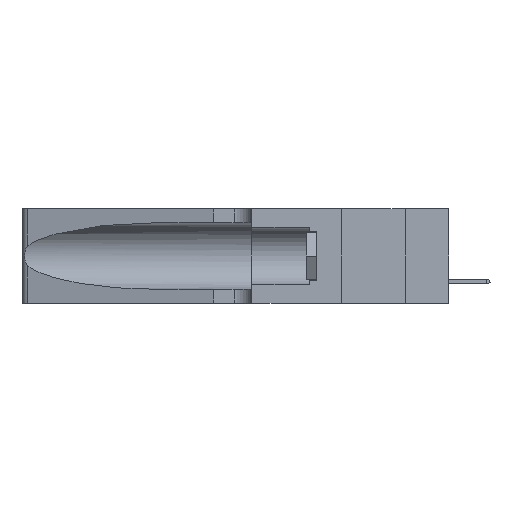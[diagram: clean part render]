
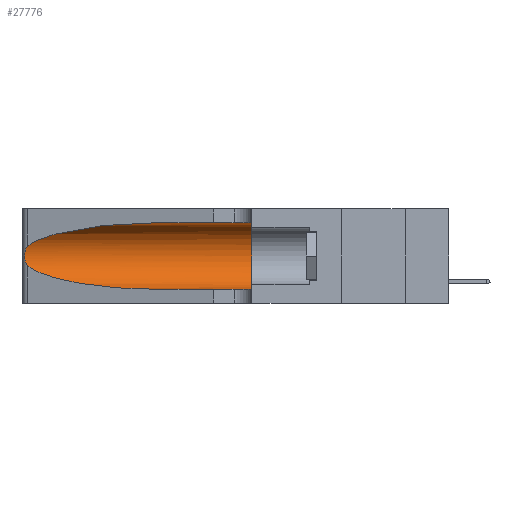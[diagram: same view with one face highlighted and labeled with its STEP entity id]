
A CAD part, left-side view. The second image highlights one B-rep face of the part: STEP entity #27776.
In plain terms, the highlighted cylindrical face has radius 3.308 mm (diameter 6.617 mm), a partial arc.
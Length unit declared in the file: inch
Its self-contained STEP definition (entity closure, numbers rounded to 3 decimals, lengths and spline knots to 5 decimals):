
#240 = VERTEX_POINT ( 'NONE', #22419 ) ;
#779 = CARTESIAN_POINT ( 'NONE',  ( 0.1305, 1.61858, 0.31525 ) ) ;
#993 = LINE ( 'NONE', #779, #8944 ) ;
#1124 = DIRECTION ( 'NONE',  ( 0., -1., 0. ) ) ;
#1543 = DIRECTION ( 'NONE',  ( 0., 0., 1. ) ) ;
#1784 = CARTESIAN_POINT ( 'NONE',  ( 0.25789, 1.23486, 0.15765 ) ) ;
#2504 = AXIS2_PLACEMENT_3D ( 'NONE', #30883, #9723, #1543 ) ;
#3566 = VERTEX_POINT ( 'NONE', #3942 ) ;
#3942 = CARTESIAN_POINT ( 'NONE',  ( 0.1305, 0.35, 0.05475 ) ) ;
#4253 = CARTESIAN_POINT ( 'NONE',  ( 0.25639, 1.23184, 0.21858 ) ) ;
#4549 = CARTESIAN_POINT ( 'NONE',  ( 0.18966, 0.96281, 0.31525 ) ) ;
#5042 = CARTESIAN_POINT ( 'NONE',  ( 0.2373, 1.15595, 0.08982 ) ) ;
#5428 = EDGE_CURVE ( 'NONE', #18067, #3566, #24555, .T. ) ;
#7059 = VERTEX_POINT ( 'NONE', #33663 ) ;
#8215 =( BOUNDED_CURVE ( )  B_SPLINE_CURVE ( 3, ( #15352, #5042, #10431, #34454 ),
 .UNSPECIFIED., .F., .T. ) 
 B_SPLINE_CURVE_WITH_KNOTS ( ( 4, 4 ),
 ( 3.44316, 4.71239 ),
 .UNSPECIFIED. ) 
 CURVE ( )  GEOMETRIC_REPRESENTATION_ITEM ( )  RATIONAL_B_SPLINE_CURVE ( ( 1., 0.87, 0.87, 1. ) ) 
 REPRESENTATION_ITEM ( '' )  );
#8944 = VECTOR ( 'NONE', #22299, 39.37008 ) ;
#9069 = DIRECTION ( 'NONE',  ( 0., 0., -1. ) ) ;
#9390 = CARTESIAN_POINT ( 'NONE',  ( 0.25854, 1.2359, 0.20912 ) ) ;
#9656 = DIRECTION ( 'NONE',  ( 0., -1., 0. ) ) ;
#9689 = CARTESIAN_POINT ( 'NONE',  ( 0.2373, 1.15595, 0.28018 ) ) ;
#9723 = DIRECTION ( 'NONE',  ( 0., 1., 0. ) ) ;
#9742 = CARTESIAN_POINT ( 'NONE',  ( 0.25639, 1.23186, 0.15144 ) ) ;
#9858 = CARTESIAN_POINT ( 'NONE',  ( 0.25487, 1.22718, 0.14631 ) ) ;
#9927 = CARTESIAN_POINT ( 'NONE',  ( 0.25487, 1.22718, 0.22369 ) ) ;
#10431 = CARTESIAN_POINT ( 'NONE',  ( 0.18966, 0.96281, 0.05475 ) ) ;
#10517 = ORIENTED_EDGE ( 'NONE', *, *, #25509, .T. ) ;
#11369 = CYLINDRICAL_SURFACE ( 'NONE', #30823, 0.13025 ) ;
#11950 = EDGE_CURVE ( 'NONE', #7059, #240, #20709, .T. ) ;
#12295 = CARTESIAN_POINT ( 'NONE',  ( 0.1305, 0.72297, 0.31525 ) ) ;
#12446 = ORIENTED_EDGE ( 'NONE', *, *, #11950, .T. ) ;
#12728 = VERTEX_POINT ( 'NONE', #17952 ) ;
#14496 = EDGE_CURVE ( 'NONE', #12728, #7059, #25820, .T. ) ;
#15352 = CARTESIAN_POINT ( 'NONE',  ( 0.25487, 1.22718, 0.14631 ) ) ;
#16050 = ORIENTED_EDGE ( 'NONE', *, *, #5428, .F. ) ;
#16152 = ORIENTED_EDGE ( 'NONE', *, *, #25764, .F. ) ;
#17034 = CARTESIAN_POINT ( 'NONE',  ( 0.1305, 1.61858, 0.185 ) ) ;
#17288 = ORIENTED_EDGE ( 'NONE', *, *, #18396, .T. ) ;
#17952 = CARTESIAN_POINT ( 'NONE',  ( 0.1305, 0.72297, 0.31525 ) ) ;
#18067 = VERTEX_POINT ( 'NONE', #29115 ) ;
#18165 = LINE ( 'NONE', #33691, #22287 ) ;
#18396 = EDGE_CURVE ( 'NONE', #24721, #3566, #18165, .T. ) ;
#20376 = CARTESIAN_POINT ( 'NONE',  ( 0.25487, 1.22718, 0.22369 ) ) ;
#20709 = B_SPLINE_CURVE_WITH_KNOTS ( 'NONE', 3,
 ( #20376, #25865, #4253, #25505, #9390, #23046, #28556, #25749, #22933, #25383, #1784, #9742, #28082, #9858 ),
 .UNSPECIFIED., .F., .F.,
 ( 4, 2, 2, 2, 2, 2, 4 ),
 ( 0., 0.00027, 0.00053, 0.00107, 0.0016, 0.00187, 0.00214 ),
 .UNSPECIFIED. ) ;
#20992 = ORIENTED_EDGE ( 'NONE', *, *, #14496, .T. ) ;
#21485 = EDGE_LOOP ( 'NONE', ( #20992, #12446, #10517, #17288, #16050, #16152 ) ) ;
#22287 = VECTOR ( 'NONE', #9656, 39.37008 ) ;
#22299 = DIRECTION ( 'NONE',  ( 0., -1., 0. ) ) ;
#22419 = CARTESIAN_POINT ( 'NONE',  ( 0.25487, 1.22718, 0.14631 ) ) ;
#22933 = CARTESIAN_POINT ( 'NONE',  ( 0.26017, 1.23833, 0.17102 ) ) ;
#23046 = CARTESIAN_POINT ( 'NONE',  ( 0.26018, 1.23835, 0.19895 ) ) ;
#24555 = CIRCLE ( 'NONE', #2504, 0.13025 ) ;
#24721 = VERTEX_POINT ( 'NONE', #31887 ) ;
#25383 = CARTESIAN_POINT ( 'NONE',  ( 0.25856, 1.23593, 0.16098 ) ) ;
#25505 = CARTESIAN_POINT ( 'NONE',  ( 0.25787, 1.23484, 0.2124 ) ) ;
#25509 = EDGE_CURVE ( 'NONE', #240, #24721, #8215, .T. ) ;
#25749 = CARTESIAN_POINT ( 'NONE',  ( 0.26075, 1.23896, 0.178 ) ) ;
#25764 = EDGE_CURVE ( 'NONE', #12728, #18067, #993, .T. ) ;
#25820 =( BOUNDED_CURVE ( )  B_SPLINE_CURVE ( 3, ( #12295, #4549, #9689, #9927 ),
 .UNSPECIFIED., .F., .T. ) 
 B_SPLINE_CURVE_WITH_KNOTS ( ( 4, 4 ),
 ( 1.5708, 2.84003 ),
 .UNSPECIFIED. ) 
 CURVE ( )  GEOMETRIC_REPRESENTATION_ITEM ( )  RATIONAL_B_SPLINE_CURVE ( ( 1., 0.87, 0.87, 1. ) ) 
 REPRESENTATION_ITEM ( '' )  );
#25865 = CARTESIAN_POINT ( 'NONE',  ( 0.25555, 1.22994, 0.2215 ) ) ;
#27776 = ADVANCED_FACE ( 'NONE', ( #31022 ), #11369, .F. ) ;
#28082 = CARTESIAN_POINT ( 'NONE',  ( 0.25555, 1.22993, 0.14849 ) ) ;
#28556 = CARTESIAN_POINT ( 'NONE',  ( 0.26075, 1.23896, 0.19203 ) ) ;
#29115 = CARTESIAN_POINT ( 'NONE',  ( 0.1305, 0.35, 0.31525 ) ) ;
#30823 = AXIS2_PLACEMENT_3D ( 'NONE', #17034, #1124, #9069 ) ;
#30883 = CARTESIAN_POINT ( 'NONE',  ( 0.1305, 0.35, 0.185 ) ) ;
#31022 = FACE_OUTER_BOUND ( 'NONE', #21485, .T. ) ;
#31887 = CARTESIAN_POINT ( 'NONE',  ( 0.1305, 0.72297, 0.05475 ) ) ;
#33663 = CARTESIAN_POINT ( 'NONE',  ( 0.25487, 1.22718, 0.22369 ) ) ;
#33691 = CARTESIAN_POINT ( 'NONE',  ( 0.1305, 1.61858, 0.05475 ) ) ;
#34454 = CARTESIAN_POINT ( 'NONE',  ( 0.1305, 0.72297, 0.05475 ) ) ;
